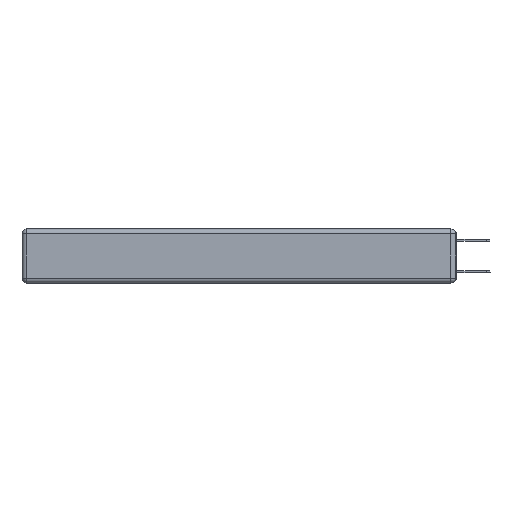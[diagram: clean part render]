
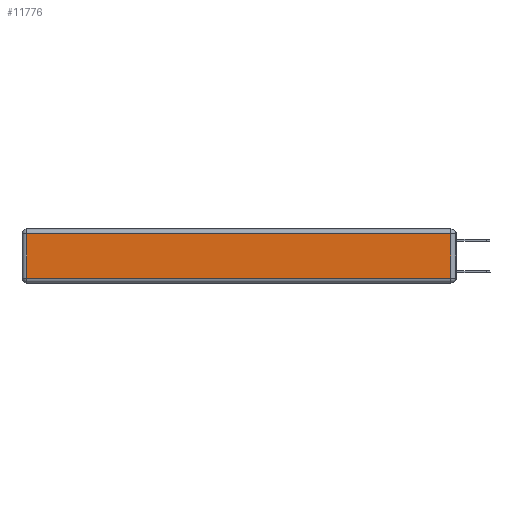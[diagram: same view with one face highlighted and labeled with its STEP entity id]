
A CAD part, left-side view. The second image highlights one B-rep face of the part: STEP entity #11776.
In plain terms, the highlighted planar face has unit normal (-1, 0, 0).
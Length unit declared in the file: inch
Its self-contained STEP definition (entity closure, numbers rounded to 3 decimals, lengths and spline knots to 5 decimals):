
#358 = LINE ( 'NONE', #13832, #977 ) ;
#637 = VECTOR ( 'NONE', #8287, 39.37008 ) ;
#977 = VECTOR ( 'NONE', #7797, 39.37008 ) ;
#1394 = EDGE_CURVE ( 'NONE', #7163, #9540, #8189, .T. ) ;
#1796 = EDGE_CURVE ( 'NONE', #4239, #7737, #358, .T. ) ;
#2767 = CARTESIAN_POINT ( 'NONE',  ( 0., 2.72, -0.313 ) ) ;
#2794 = CARTESIAN_POINT ( 'NONE',  ( 0., 0., -0.343 ) ) ;
#2825 = EDGE_CURVE ( 'NONE', #9540, #4239, #14424, .T. ) ;
#3098 = AXIS2_PLACEMENT_3D ( 'NONE', #2794, #6429, #14829 ) ;
#4239 = VERTEX_POINT ( 'NONE', #2767 ) ;
#4713 = CARTESIAN_POINT ( 'NONE',  ( 0., 2.75, -0.03 ) ) ;
#4760 = DIRECTION ( 'NONE',  ( 0., 0., -1. ) ) ;
#4950 = EDGE_CURVE ( 'NONE', #7737, #7163, #14317, .T. ) ;
#5107 = VECTOR ( 'NONE', #4760, 39.37008 ) ;
#6429 = DIRECTION ( 'NONE',  ( -1., 0., 0. ) ) ;
#6578 = PLANE ( 'NONE',  #3098 ) ;
#7163 = VERTEX_POINT ( 'NONE', #8490 ) ;
#7737 = VERTEX_POINT ( 'NONE', #13003 ) ;
#7797 = DIRECTION ( 'NONE',  ( 0., -1., 0. ) ) ;
#8189 = LINE ( 'NONE', #4713, #13305 ) ;
#8287 = DIRECTION ( 'NONE',  ( 0., 0., 1. ) ) ;
#8367 = CARTESIAN_POINT ( 'NONE',  ( 0., 0.03, -0.343 ) ) ;
#8490 = CARTESIAN_POINT ( 'NONE',  ( 0., 0.03, -0.03 ) ) ;
#9540 = VERTEX_POINT ( 'NONE', #13539 ) ;
#10138 = FACE_OUTER_BOUND ( 'NONE', #14279, .T. ) ;
#10885 = CARTESIAN_POINT ( 'NONE',  ( 0., 2.72, -0.343 ) ) ;
#10968 = ORIENTED_EDGE ( 'NONE', *, *, #1394, .T. ) ;
#11776 = ADVANCED_FACE ( 'NONE', ( #10138 ), #6578, .T. ) ;
#12314 = ORIENTED_EDGE ( 'NONE', *, *, #4950, .T. ) ;
#13003 = CARTESIAN_POINT ( 'NONE',  ( 0., 0.03, -0.313 ) ) ;
#13305 = VECTOR ( 'NONE', #15154, 39.37008 ) ;
#13539 = CARTESIAN_POINT ( 'NONE',  ( 0., 2.72, -0.03 ) ) ;
#13714 = ORIENTED_EDGE ( 'NONE', *, *, #2825, .T. ) ;
#13832 = CARTESIAN_POINT ( 'NONE',  ( 0., 0., -0.313 ) ) ;
#14279 = EDGE_LOOP ( 'NONE', ( #14589, #12314, #10968, #13714 ) ) ;
#14317 = LINE ( 'NONE', #8367, #637 ) ;
#14424 = LINE ( 'NONE', #10885, #5107 ) ;
#14589 = ORIENTED_EDGE ( 'NONE', *, *, #1796, .T. ) ;
#14829 = DIRECTION ( 'NONE',  ( 0., 0., 1. ) ) ;
#15154 = DIRECTION ( 'NONE',  ( 0., 1., 0. ) ) ;
